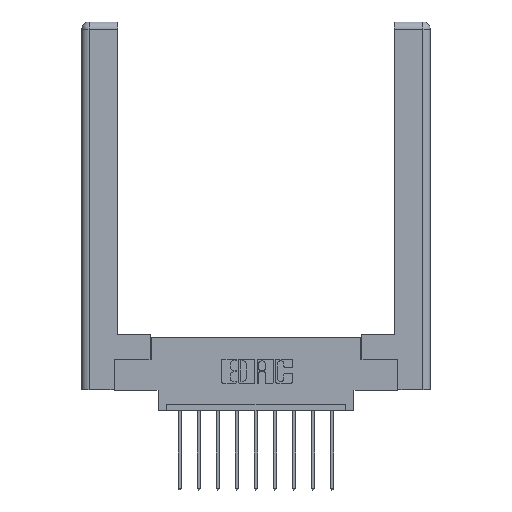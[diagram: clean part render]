
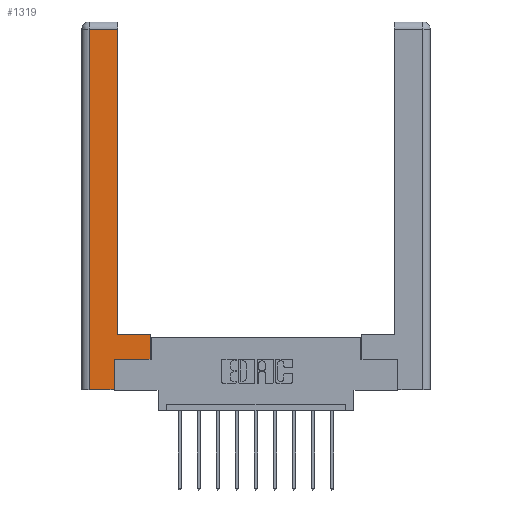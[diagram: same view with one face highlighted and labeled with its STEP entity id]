
A CAD part, top view. The second image highlights one B-rep face of the part: STEP entity #1319.
In plain terms, the highlighted planar face has unit normal (0, 0, 1).
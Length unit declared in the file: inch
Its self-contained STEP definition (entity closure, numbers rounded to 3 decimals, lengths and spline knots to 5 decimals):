
#79 = DIRECTION ( 'NONE',  ( 0., 0., -1. ) ) ;
#225 = VERTEX_POINT ( 'NONE', #7643 ) ;
#240 = LINE ( 'NONE', #9828, #8879 ) ;
#851 = CARTESIAN_POINT ( 'NONE',  ( 0.0615, 0., 0. ) ) ;
#939 = CARTESIAN_POINT ( 'NONE',  ( 0.295, 2.94, 0. ) ) ;
#1047 = EDGE_CURVE ( 'NONE', #2181, #7883, #12559, .T. ) ;
#1069 = ORIENTED_EDGE ( 'NONE', *, *, #4097, .T. ) ;
#1253 = VECTOR ( 'NONE', #11905, 39.37008 ) ;
#1319 = ADVANCED_FACE ( 'NONE', ( #7763 ), #1468, .F. ) ;
#1420 = CARTESIAN_POINT ( 'NONE',  ( 0.265, 0., 0. ) ) ;
#1468 = PLANE ( 'NONE',  #1763 ) ;
#1555 = DIRECTION ( 'NONE',  ( 1., 0., 0. ) ) ;
#1763 = AXIS2_PLACEMENT_3D ( 'NONE', #7618, #79, #11847 ) ;
#2018 = VECTOR ( 'NONE', #1555, 39.37008 ) ;
#2028 = VECTOR ( 'NONE', #7260, 39.37008 ) ;
#2097 = CARTESIAN_POINT ( 'NONE',  ( 0.0615, 2.94, 0. ) ) ;
#2130 = ORIENTED_EDGE ( 'NONE', *, *, #11656, .T. ) ;
#2143 = VERTEX_POINT ( 'NONE', #9228 ) ;
#2181 = VERTEX_POINT ( 'NONE', #5864 ) ;
#2557 = VERTEX_POINT ( 'NONE', #5672 ) ;
#2881 = VECTOR ( 'NONE', #9546, 39.37008 ) ;
#3007 = CARTESIAN_POINT ( 'NONE',  ( 0.295, 3., 0. ) ) ;
#3430 = EDGE_CURVE ( 'NONE', #225, #3916, #240, .T. ) ;
#3663 = ORIENTED_EDGE ( 'NONE', *, *, #5712, .T. ) ;
#3664 = ORIENTED_EDGE ( 'NONE', *, *, #1047, .T. ) ;
#3724 = EDGE_CURVE ( 'NONE', #2557, #4450, #4861, .T. ) ;
#3916 = VERTEX_POINT ( 'NONE', #6042 ) ;
#4097 = EDGE_CURVE ( 'NONE', #2143, #225, #13167, .T. ) ;
#4329 = VECTOR ( 'NONE', #4952, 39.37008 ) ;
#4450 = VERTEX_POINT ( 'NONE', #939 ) ;
#4861 = LINE ( 'NONE', #3007, #2028 ) ;
#4952 = DIRECTION ( 'NONE',  ( 0., -1., 0. ) ) ;
#5672 = CARTESIAN_POINT ( 'NONE',  ( 0.295, 0.45, 0. ) ) ;
#5675 = VECTOR ( 'NONE', #13661, 39.37008 ) ;
#5712 = EDGE_CURVE ( 'NONE', #7883, #2557, #11808, .T. ) ;
#5811 = CARTESIAN_POINT ( 'NONE',  ( 0.565, 0.45, 0. ) ) ;
#5864 = CARTESIAN_POINT ( 'NONE',  ( 0.565, 0.245, 0. ) ) ;
#6041 = VERTEX_POINT ( 'NONE', #10543 ) ;
#6042 = CARTESIAN_POINT ( 'NONE',  ( 0.265, 0.245, 0. ) ) ;
#6738 = EDGE_CURVE ( 'NONE', #3916, #2181, #12993, .T. ) ;
#6881 = EDGE_CURVE ( 'NONE', #6041, #2143, #10004, .T. ) ;
#7260 = DIRECTION ( 'NONE',  ( 0., 1., 0. ) ) ;
#7352 = EDGE_LOOP ( 'NONE', ( #11620, #2130, #13633, #1069, #8663, #8963, #3664, #3663 ) ) ;
#7618 = CARTESIAN_POINT ( 'NONE',  ( 0., 0., 0. ) ) ;
#7643 = CARTESIAN_POINT ( 'NONE',  ( 0.265, 0., 0. ) ) ;
#7763 = FACE_OUTER_BOUND ( 'NONE', #7352, .T. ) ;
#7883 = VERTEX_POINT ( 'NONE', #5811 ) ;
#8663 = ORIENTED_EDGE ( 'NONE', *, *, #3430, .T. ) ;
#8879 = VECTOR ( 'NONE', #12024, 39.37008 ) ;
#8963 = ORIENTED_EDGE ( 'NONE', *, *, #6738, .T. ) ;
#9228 = CARTESIAN_POINT ( 'NONE',  ( 0.0615, 0., 0. ) ) ;
#9324 = CARTESIAN_POINT ( 'NONE',  ( 0.565, 0.245, 0. ) ) ;
#9460 = CARTESIAN_POINT ( 'NONE',  ( 0.295, 0.45, 0. ) ) ;
#9546 = DIRECTION ( 'NONE',  ( -1., 0., 0. ) ) ;
#9828 = CARTESIAN_POINT ( 'NONE',  ( 0.265, 0.245, 0. ) ) ;
#10004 = LINE ( 'NONE', #851, #4329 ) ;
#10543 = CARTESIAN_POINT ( 'NONE',  ( 0.0615, 2.94, 0. ) ) ;
#11620 = ORIENTED_EDGE ( 'NONE', *, *, #3724, .T. ) ;
#11656 = EDGE_CURVE ( 'NONE', #4450, #6041, #12051, .T. ) ;
#11808 = LINE ( 'NONE', #9460, #5675 ) ;
#11847 = DIRECTION ( 'NONE',  ( -1., 0., 0. ) ) ;
#11905 = DIRECTION ( 'NONE',  ( 0., 1., 0. ) ) ;
#12024 = DIRECTION ( 'NONE',  ( 0., 1., 0. ) ) ;
#12051 = LINE ( 'NONE', #2097, #2881 ) ;
#12195 = VECTOR ( 'NONE', #13727, 39.37008 ) ;
#12559 = LINE ( 'NONE', #13104, #1253 ) ;
#12993 = LINE ( 'NONE', #9324, #12195 ) ;
#13104 = CARTESIAN_POINT ( 'NONE',  ( 0.565, 0.45, 0. ) ) ;
#13167 = LINE ( 'NONE', #1420, #2018 ) ;
#13633 = ORIENTED_EDGE ( 'NONE', *, *, #6881, .T. ) ;
#13661 = DIRECTION ( 'NONE',  ( -1., 0., 0. ) ) ;
#13727 = DIRECTION ( 'NONE',  ( 1., 0., 0. ) ) ;
